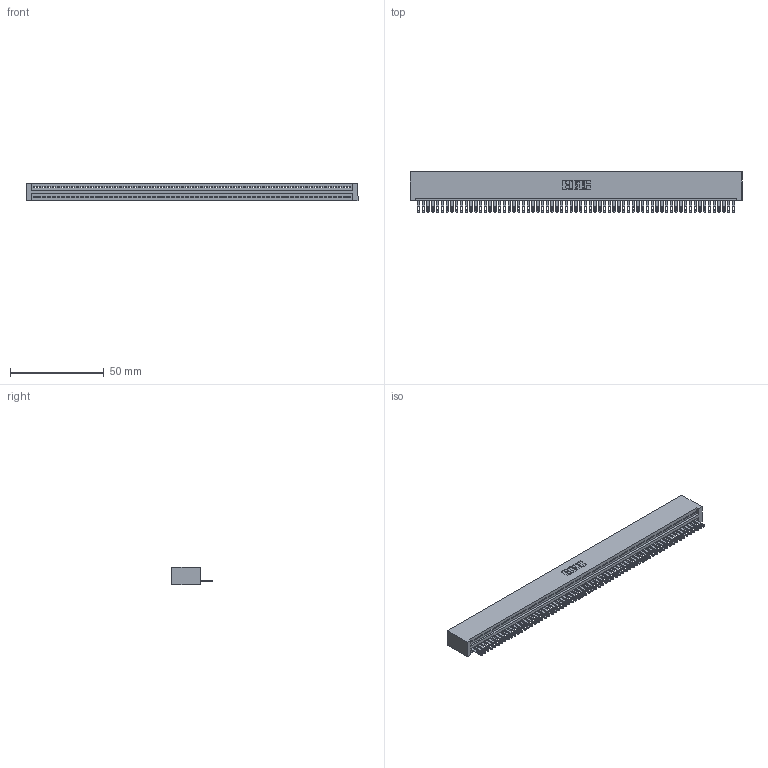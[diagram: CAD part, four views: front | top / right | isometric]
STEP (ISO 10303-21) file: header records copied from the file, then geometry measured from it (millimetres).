
FILE_DESCRIPTION (( 'STEP AP203' ), '1' );
FILE_NAME ('345-067-500-101.STEP', '2019-10-11T23:23:46', ( '' ), ( '' ), 'SwSTEP 2.0', 'SolidWorks 2016', '' );
FILE_SCHEMA (( 'CONFIG_CONTROL_DESIGN' ));
Length unit declared in the file: inch
Products named in the file (3): 345 Part_No Mounting Lugs; 345-067-500-101; 345-292-001_345-293-100
Assembly tree (68 placements, depth 2):
  345-067-500-101
    345 Part_No Mounting Lugs
    345-292-001_345-293-100  x67
Bounding box: 176.78 x 21.51 x 9.4 mm (x, y, z)
Volume: 17621.7 mm3; surface area: 24098.1 mm2
Topology: 68 solids, 68 shells, 3736 faces, 11573 edges, 7714 vertices
Faces by surface type: plane 2354, cylinder 1382
Entity records: 46713 total; most frequent: ORIENTED_EDGE 8098, CARTESIAN_POINT 8097, DIRECTION 7031, EDGE_CURVE 4049, LINE 3653, VECTOR 3653, VERTEX_POINT 2698, AXIS2_PLACEMENT_3D 1689
